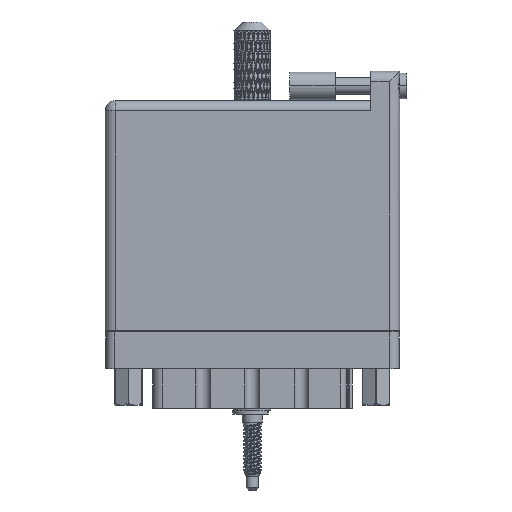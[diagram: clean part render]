
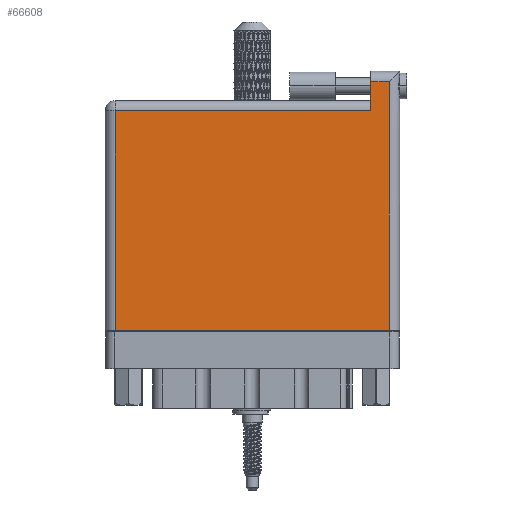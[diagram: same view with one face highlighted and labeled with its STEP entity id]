
A CAD part, front view. The second image highlights one B-rep face of the part: STEP entity #66608.
In plain terms, the highlighted face is planar.
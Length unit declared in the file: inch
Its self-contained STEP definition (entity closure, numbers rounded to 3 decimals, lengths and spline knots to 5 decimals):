
#235 = CARTESIAN_POINT ( 'NONE',  ( 1.811, 1.766, 0. ) ) ;
#2384 = EDGE_CURVE ( 'NONE', #21257, #16721, #67635, .T. ) ;
#3494 = EDGE_CURVE ( 'NONE', #40468, #21257, #21630, .T. ) ;
#5044 = CARTESIAN_POINT ( 'NONE',  ( 1.938, 1.766, 0. ) ) ;
#8825 = LINE ( 'NONE', #30422, #86977 ) ;
#12130 = EDGE_CURVE ( 'NONE', #14824, #40468, #39322, .T. ) ;
#14824 = VERTEX_POINT ( 'NONE', #105580 ) ;
#15579 = VERTEX_POINT ( 'NONE', #62078 ) ;
#16362 = VECTOR ( 'NONE', #32277, 39.37008 ) ;
#16721 = VERTEX_POINT ( 'NONE', #60557 ) ;
#19353 = EDGE_LOOP ( 'NONE', ( #49263, #105073, #95349, #50256, #36291, #46736 ) ) ;
#19475 = VECTOR ( 'NONE', #27495, 39.37008 ) ;
#19932 = CARTESIAN_POINT ( 'NONE',  ( 0., 0., 0. ) ) ;
#21257 = VERTEX_POINT ( 'NONE', #37071 ) ;
#21630 = LINE ( 'NONE', #19932, #29782 ) ;
#24057 = CARTESIAN_POINT ( 'NONE',  ( 0., 1.566, 0. ) ) ;
#25887 = DIRECTION ( 'NONE',  ( 0., -1., 0. ) ) ;
#27495 = DIRECTION ( 'NONE',  ( -1., 0., 0. ) ) ;
#29782 = VECTOR ( 'NONE', #63259, 39.37008 ) ;
#30422 = CARTESIAN_POINT ( 'NONE',  ( 0., 1.496, 0. ) ) ;
#32277 = DIRECTION ( 'NONE',  ( 0., -1., 0. ) ) ;
#32376 = DIRECTION ( 'NONE',  ( -1., 0., 0. ) ) ;
#35725 = LINE ( 'NONE', #70026, #19475 ) ;
#36291 = ORIENTED_EDGE ( 'NONE', *, *, #100695, .T. ) ;
#37071 = CARTESIAN_POINT ( 'NONE',  ( 1.938, 0., 0. ) ) ;
#39322 = LINE ( 'NONE', #110813, #16362 ) ;
#40468 = VERTEX_POINT ( 'NONE', #45344 ) ;
#40644 = VERTEX_POINT ( 'NONE', #55296 ) ;
#45344 = CARTESIAN_POINT ( 'NONE',  ( 0.07, 0., 0. ) ) ;
#46736 = ORIENTED_EDGE ( 'NONE', *, *, #12130, .T. ) ;
#49263 = ORIENTED_EDGE ( 'NONE', *, *, #3494, .T. ) ;
#50256 = ORIENTED_EDGE ( 'NONE', *, *, #97874, .T. ) ;
#54724 = AXIS2_PLACEMENT_3D ( 'NONE', #24057, #92176, #32376 ) ;
#55296 = CARTESIAN_POINT ( 'NONE',  ( 1.811, 1.496, 0. ) ) ;
#57957 = VECTOR ( 'NONE', #25887, 39.37008 ) ;
#60557 = CARTESIAN_POINT ( 'NONE',  ( 1.938, 1.696, 0. ) ) ;
#62078 = CARTESIAN_POINT ( 'NONE',  ( 1.811, 1.696, 0. ) ) ;
#63259 = DIRECTION ( 'NONE',  ( 1., 0., 0. ) ) ;
#66608 = ADVANCED_FACE ( 'NONE', ( #103715 ), #83886, .F. ) ;
#67635 = LINE ( 'NONE', #5044, #89132 ) ;
#70026 = CARTESIAN_POINT ( 'NONE',  ( 0., 1.696, 0. ) ) ;
#83886 = PLANE ( 'NONE',  #54724 ) ;
#84690 = LINE ( 'NONE', #235, #57957 ) ;
#86977 = VECTOR ( 'NONE', #89876, 39.37008 ) ;
#89132 = VECTOR ( 'NONE', #99222, 39.37008 ) ;
#89876 = DIRECTION ( 'NONE',  ( -1., 0., 0. ) ) ;
#92176 = DIRECTION ( 'NONE',  ( 0., 0., -1. ) ) ;
#95349 = ORIENTED_EDGE ( 'NONE', *, *, #101685, .T. ) ;
#97874 = EDGE_CURVE ( 'NONE', #15579, #40644, #84690, .T. ) ;
#99222 = DIRECTION ( 'NONE',  ( 0., 1., 0. ) ) ;
#100695 = EDGE_CURVE ( 'NONE', #40644, #14824, #8825, .T. ) ;
#101685 = EDGE_CURVE ( 'NONE', #16721, #15579, #35725, .T. ) ;
#103715 = FACE_OUTER_BOUND ( 'NONE', #19353, .T. ) ;
#105073 = ORIENTED_EDGE ( 'NONE', *, *, #2384, .T. ) ;
#105580 = CARTESIAN_POINT ( 'NONE',  ( 0.07, 1.496, 0. ) ) ;
#110813 = CARTESIAN_POINT ( 'NONE',  ( 0.07, 0., 0. ) ) ;
